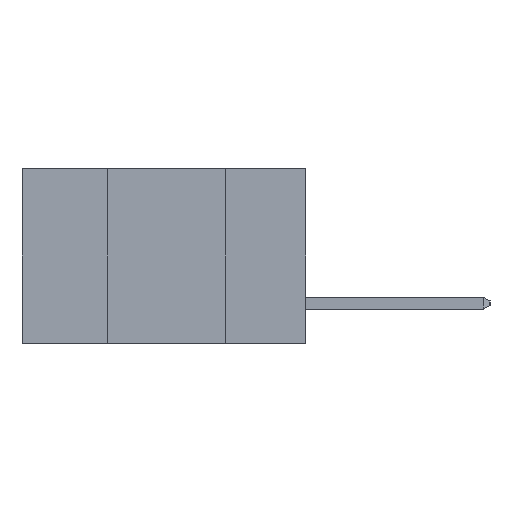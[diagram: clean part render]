
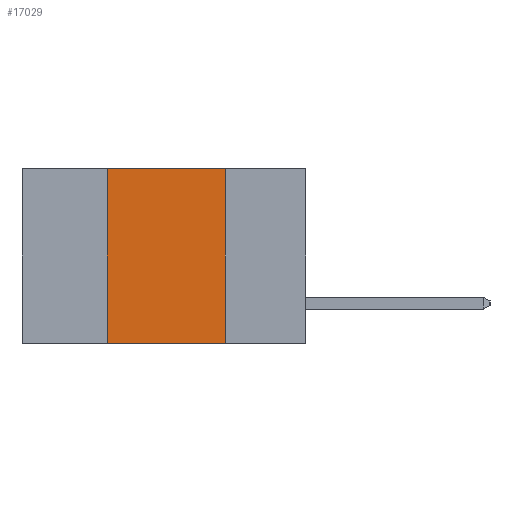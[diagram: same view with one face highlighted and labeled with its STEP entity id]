
A CAD part, left-side view. The second image highlights one B-rep face of the part: STEP entity #17029.
In plain terms, the highlighted planar face has unit normal (-1, 0, 0).
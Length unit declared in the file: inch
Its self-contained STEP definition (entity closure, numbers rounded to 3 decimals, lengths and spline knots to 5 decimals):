
#221 = CARTESIAN_POINT ( 'NONE',  ( 0., 0.6, 0. ) ) ;
#343 = AXIS2_PLACEMENT_3D ( 'NONE', #221, #13377, #3580 ) ;
#753 = EDGE_CURVE ( 'NONE', #14390, #9969, #6972, .T. ) ;
#1182 = CARTESIAN_POINT ( 'NONE',  ( 0., 0.42, 0. ) ) ;
#1320 = CARTESIAN_POINT ( 'NONE',  ( 0., 0.17, 0. ) ) ;
#2232 = ORIENTED_EDGE ( 'NONE', *, *, #7879, .F. ) ;
#2998 = DIRECTION ( 'NONE',  ( 0., 0., -1. ) ) ;
#3580 = DIRECTION ( 'NONE',  ( 0., 0., -1. ) ) ;
#4504 = VECTOR ( 'NONE', #2998, 39.37008 ) ;
#5968 = VERTEX_POINT ( 'NONE', #1182 ) ;
#6613 = ORIENTED_EDGE ( 'NONE', *, *, #19198, .F. ) ;
#6972 = LINE ( 'NONE', #20472, #15092 ) ;
#7879 = EDGE_CURVE ( 'NONE', #5968, #14767, #15899, .T. ) ;
#8407 = CARTESIAN_POINT ( 'NONE',  ( 0., 0.17, -0.37 ) ) ;
#8914 = DIRECTION ( 'NONE',  ( 0., -1., 0. ) ) ;
#9541 = EDGE_LOOP ( 'NONE', ( #10505, #2232, #6613, #15731 ) ) ;
#9918 = LINE ( 'NONE', #1320, #4504 ) ;
#9969 = VERTEX_POINT ( 'NONE', #8407 ) ;
#10505 = ORIENTED_EDGE ( 'NONE', *, *, #15645, .F. ) ;
#10929 = CARTESIAN_POINT ( 'NONE',  ( 0., 0.42, 0. ) ) ;
#11403 = CARTESIAN_POINT ( 'NONE',  ( 0., 0.42, -0.37 ) ) ;
#11798 = PLANE ( 'NONE',  #343 ) ;
#12529 = DIRECTION ( 'NONE',  ( 0., 0., 1. ) ) ;
#13283 = CARTESIAN_POINT ( 'NONE',  ( 0., 0.6, 0. ) ) ;
#13377 = DIRECTION ( 'NONE',  ( 1., 0., 0. ) ) ;
#14353 = FACE_OUTER_BOUND ( 'NONE', #9541, .T. ) ;
#14390 = VERTEX_POINT ( 'NONE', #11403 ) ;
#14767 = VERTEX_POINT ( 'NONE', #15474 ) ;
#15092 = VECTOR ( 'NONE', #20698, 39.37008 ) ;
#15474 = CARTESIAN_POINT ( 'NONE',  ( 0., 0.17, 0. ) ) ;
#15645 = EDGE_CURVE ( 'NONE', #14767, #9969, #9918, .T. ) ;
#15731 = ORIENTED_EDGE ( 'NONE', *, *, #753, .T. ) ;
#15899 = LINE ( 'NONE', #13283, #19562 ) ;
#16001 = VECTOR ( 'NONE', #12529, 39.37008 ) ;
#16482 = LINE ( 'NONE', #10929, #16001 ) ;
#17029 = ADVANCED_FACE ( 'NONE', ( #14353 ), #11798, .F. ) ;
#19198 = EDGE_CURVE ( 'NONE', #14390, #5968, #16482, .T. ) ;
#19562 = VECTOR ( 'NONE', #8914, 39.37008 ) ;
#20472 = CARTESIAN_POINT ( 'NONE',  ( 0., 0.6, -0.37 ) ) ;
#20698 = DIRECTION ( 'NONE',  ( 0., -1., 0. ) ) ;
